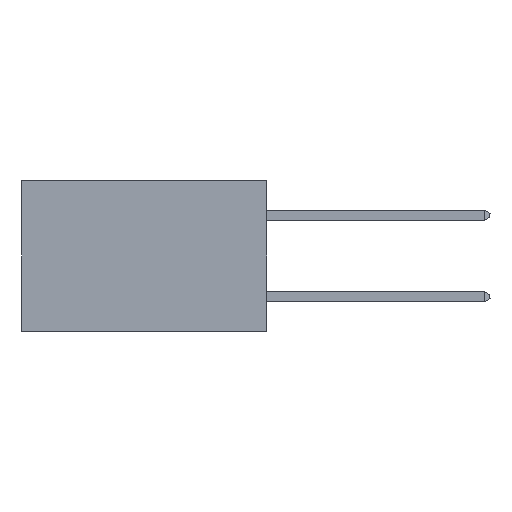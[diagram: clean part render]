
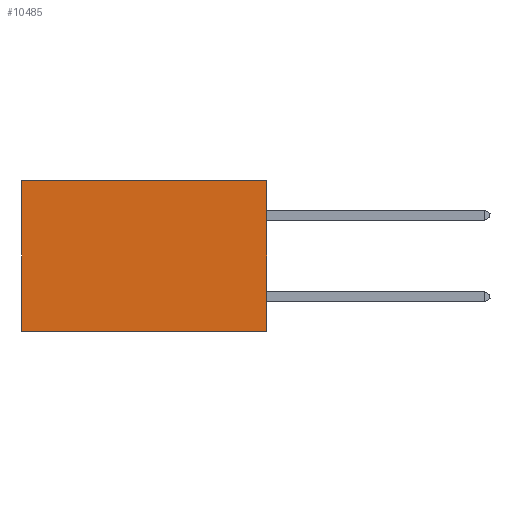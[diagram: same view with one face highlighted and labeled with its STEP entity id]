
A CAD part, left-side view. The second image highlights one B-rep face of the part: STEP entity #10485.
In plain terms, the highlighted planar face has unit normal (-1, 0, 0).
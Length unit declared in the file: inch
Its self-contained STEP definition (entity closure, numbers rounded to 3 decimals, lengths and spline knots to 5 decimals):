
#648 = DIRECTION ( 'NONE',  ( 1., 0., 0. ) ) ;
#1657 = CARTESIAN_POINT ( 'NONE',  ( 0.2875, 0., -0.37 ) ) ;
#2438 = VECTOR ( 'NONE', #13780, 39.37008 ) ;
#2590 = VERTEX_POINT ( 'NONE', #19134 ) ;
#2770 = LINE ( 'NONE', #16285, #15992 ) ;
#4217 = PLANE ( 'NONE',  #20757 ) ;
#5444 = EDGE_CURVE ( 'NONE', #13799, #9476, #7725, .T. ) ;
#5551 = CARTESIAN_POINT ( 'NONE',  ( 0.2875, 0., 0. ) ) ;
#7725 = LINE ( 'NONE', #10018, #14127 ) ;
#7837 = DIRECTION ( 'NONE',  ( 0., 0., -1. ) ) ;
#9476 = VERTEX_POINT ( 'NONE', #18589 ) ;
#9938 = DIRECTION ( 'NONE',  ( 0., 0., -1. ) ) ;
#10018 = CARTESIAN_POINT ( 'NONE',  ( 0.2875, 0., 0. ) ) ;
#10485 = ADVANCED_FACE ( 'NONE', ( #16911 ), #4217, .F. ) ;
#10763 = ORIENTED_EDGE ( 'NONE', *, *, #15006, .F. ) ;
#11698 = DIRECTION ( 'NONE',  ( 0., 1., 0. ) ) ;
#12876 = VECTOR ( 'NONE', #11698, 39.37008 ) ;
#12943 = DIRECTION ( 'NONE',  ( 0., 0., -1. ) ) ;
#13403 = LINE ( 'NONE', #16639, #12876 ) ;
#13780 = DIRECTION ( 'NONE',  ( 0., 1., 0. ) ) ;
#13799 = VERTEX_POINT ( 'NONE', #5551 ) ;
#13999 = EDGE_CURVE ( 'NONE', #15506, #2590, #2770, .T. ) ;
#14120 = EDGE_CURVE ( 'NONE', #13799, #15506, #13403, .T. ) ;
#14127 = VECTOR ( 'NONE', #9938, 39.37008 ) ;
#15006 = EDGE_CURVE ( 'NONE', #9476, #2590, #15688, .T. ) ;
#15323 = ORIENTED_EDGE ( 'NONE', *, *, #14120, .T. ) ;
#15506 = VERTEX_POINT ( 'NONE', #18373 ) ;
#15688 = LINE ( 'NONE', #1657, #2438 ) ;
#15992 = VECTOR ( 'NONE', #7837, 39.37008 ) ;
#16204 = CARTESIAN_POINT ( 'NONE',  ( 0.2875, 0., 0. ) ) ;
#16285 = CARTESIAN_POINT ( 'NONE',  ( 0.2875, 0.6, 0. ) ) ;
#16639 = CARTESIAN_POINT ( 'NONE',  ( 0.2875, 0., 0. ) ) ;
#16911 = FACE_OUTER_BOUND ( 'NONE', #19252, .T. ) ;
#18214 = ORIENTED_EDGE ( 'NONE', *, *, #5444, .F. ) ;
#18373 = CARTESIAN_POINT ( 'NONE',  ( 0.2875, 0.6, 0. ) ) ;
#18589 = CARTESIAN_POINT ( 'NONE',  ( 0.2875, 0., -0.37 ) ) ;
#18625 = ORIENTED_EDGE ( 'NONE', *, *, #13999, .T. ) ;
#19134 = CARTESIAN_POINT ( 'NONE',  ( 0.2875, 0.6, -0.37 ) ) ;
#19252 = EDGE_LOOP ( 'NONE', ( #18625, #10763, #18214, #15323 ) ) ;
#20757 = AXIS2_PLACEMENT_3D ( 'NONE', #16204, #648, #12943 ) ;
